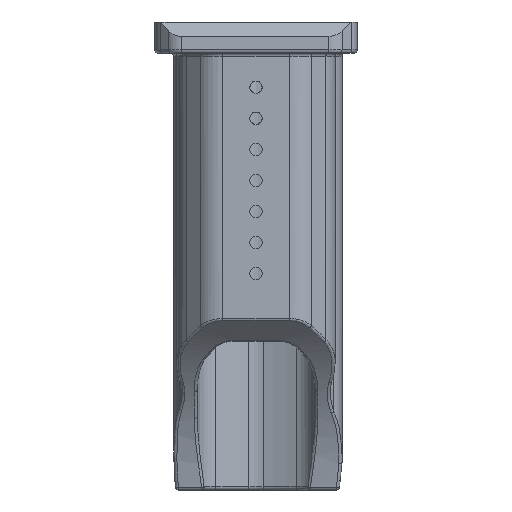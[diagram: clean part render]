
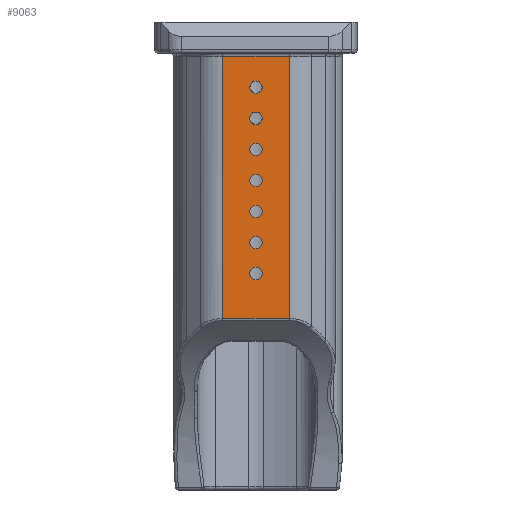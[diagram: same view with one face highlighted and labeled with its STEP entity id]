
A CAD part, front view. The second image highlights one B-rep face of the part: STEP entity #9063.
In plain terms, the highlighted planar face has unit normal (0, -1, 0).
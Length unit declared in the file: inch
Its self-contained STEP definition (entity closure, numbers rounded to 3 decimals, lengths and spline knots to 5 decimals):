
#30=FACE_BOUND('',#1518,.T.);
#31=FACE_BOUND('',#1519,.T.);
#32=FACE_BOUND('',#1520,.T.);
#33=FACE_BOUND('',#1521,.T.);
#34=FACE_BOUND('',#1522,.T.);
#35=FACE_BOUND('',#1523,.T.);
#36=FACE_BOUND('',#1524,.T.);
#308=PLANE('',#9837);
#985=FACE_OUTER_BOUND('',#1517,.T.);
#1517=EDGE_LOOP('',(#7756,#7757,#7758,#7759));
#1518=EDGE_LOOP('',(#7760,#7761));
#1519=EDGE_LOOP('',(#7762,#7763));
#1520=EDGE_LOOP('',(#7764,#7765));
#1521=EDGE_LOOP('',(#7766,#7767));
#1522=EDGE_LOOP('',(#7768,#7769));
#1523=EDGE_LOOP('',(#7770,#7771));
#1524=EDGE_LOOP('',(#7772,#7773));
#2366=LINE('',#16193,#3183);
#2373=LINE('',#16830,#3190);
#2374=LINE('',#16834,#3191);
#2375=LINE('',#16835,#3192);
#3183=VECTOR('',#11880,0.3937);
#3190=VECTOR('',#11945,0.5);
#3191=VECTOR('',#11950,0.3937);
#3192=VECTOR('',#11951,0.3937);
#3409=CIRCLE('',#9371,0.09843);
#3410=CIRCLE('',#9372,0.09843);
#3412=CIRCLE('',#9375,0.09843);
#3413=CIRCLE('',#9376,0.09843);
#3415=CIRCLE('',#9379,0.09843);
#3416=CIRCLE('',#9380,0.09843);
#3418=CIRCLE('',#9383,0.09843);
#3419=CIRCLE('',#9384,0.09843);
#3421=CIRCLE('',#9387,0.09843);
#3422=CIRCLE('',#9388,0.09843);
#3423=CIRCLE('',#9392,0.09843);
#3424=CIRCLE('',#9393,0.09843);
#3427=CIRCLE('',#9398,0.09843);
#3428=CIRCLE('',#9399,0.09843);
#3825=VERTEX_POINT('',#13624);
#3826=VERTEX_POINT('',#13625);
#3828=VERTEX_POINT('',#13632);
#3829=VERTEX_POINT('',#13633);
#3831=VERTEX_POINT('',#13640);
#3832=VERTEX_POINT('',#13641);
#3834=VERTEX_POINT('',#13648);
#3835=VERTEX_POINT('',#13649);
#3837=VERTEX_POINT('',#13656);
#3838=VERTEX_POINT('',#13657);
#3841=VERTEX_POINT('',#13666);
#3842=VERTEX_POINT('',#13667);
#3846=VERTEX_POINT('',#13678);
#3847=VERTEX_POINT('',#13679);
#4361=VERTEX_POINT('',#16170);
#4363=VERTEX_POINT('',#16191);
#4395=VERTEX_POINT('',#16829);
#4396=VERTEX_POINT('',#16833);
#4716=EDGE_CURVE('',#3825,#3826,#3409,.T.);
#4717=EDGE_CURVE('',#3826,#3825,#3410,.T.);
#4720=EDGE_CURVE('',#3828,#3829,#3412,.T.);
#4721=EDGE_CURVE('',#3829,#3828,#3413,.T.);
#4724=EDGE_CURVE('',#3831,#3832,#3415,.T.);
#4725=EDGE_CURVE('',#3832,#3831,#3416,.T.);
#4728=EDGE_CURVE('',#3834,#3835,#3418,.T.);
#4729=EDGE_CURVE('',#3835,#3834,#3419,.T.);
#4732=EDGE_CURVE('',#3837,#3838,#3421,.T.);
#4733=EDGE_CURVE('',#3838,#3837,#3422,.T.);
#4737=EDGE_CURVE('',#3841,#3842,#3423,.T.);
#4738=EDGE_CURVE('',#3842,#3841,#3424,.T.);
#4743=EDGE_CURVE('',#3846,#3847,#3427,.T.);
#4744=EDGE_CURVE('',#3847,#3846,#3428,.T.);
#5540=EDGE_CURVE('',#4363,#4361,#2366,.T.);
#5593=EDGE_CURVE('',#4395,#4361,#2373,.T.);
#5595=EDGE_CURVE('',#4396,#4363,#2374,.T.);
#5596=EDGE_CURVE('',#4395,#4396,#2375,.T.);
#7756=ORIENTED_EDGE('',*,*,#5540,.F.);
#7757=ORIENTED_EDGE('',*,*,#5595,.F.);
#7758=ORIENTED_EDGE('',*,*,#5596,.F.);
#7759=ORIENTED_EDGE('',*,*,#5593,.T.);
#7760=ORIENTED_EDGE('',*,*,#4716,.T.);
#7761=ORIENTED_EDGE('',*,*,#4717,.T.);
#7762=ORIENTED_EDGE('',*,*,#4720,.T.);
#7763=ORIENTED_EDGE('',*,*,#4721,.T.);
#7764=ORIENTED_EDGE('',*,*,#4724,.T.);
#7765=ORIENTED_EDGE('',*,*,#4725,.T.);
#7766=ORIENTED_EDGE('',*,*,#4728,.T.);
#7767=ORIENTED_EDGE('',*,*,#4729,.T.);
#7768=ORIENTED_EDGE('',*,*,#4732,.T.);
#7769=ORIENTED_EDGE('',*,*,#4733,.T.);
#7770=ORIENTED_EDGE('',*,*,#4737,.T.);
#7771=ORIENTED_EDGE('',*,*,#4738,.T.);
#7772=ORIENTED_EDGE('',*,*,#4743,.T.);
#7773=ORIENTED_EDGE('',*,*,#4744,.T.);
#9063=ADVANCED_FACE('',(#985,#30,#31,#32,#33,#34,#35,#36),#308,.T.);
#9371=AXIS2_PLACEMENT_3D('',#13626,#10412,#10413);
#9372=AXIS2_PLACEMENT_3D('',#13627,#10414,#10415);
#9375=AXIS2_PLACEMENT_3D('',#13634,#10421,#10422);
#9376=AXIS2_PLACEMENT_3D('',#13635,#10423,#10424);
#9379=AXIS2_PLACEMENT_3D('',#13642,#10430,#10431);
#9380=AXIS2_PLACEMENT_3D('',#13643,#10432,#10433);
#9383=AXIS2_PLACEMENT_3D('',#13650,#10439,#10440);
#9384=AXIS2_PLACEMENT_3D('',#13651,#10441,#10442);
#9387=AXIS2_PLACEMENT_3D('',#13658,#10448,#10449);
#9388=AXIS2_PLACEMENT_3D('',#13659,#10450,#10451);
#9392=AXIS2_PLACEMENT_3D('',#13668,#10459,#10460);
#9393=AXIS2_PLACEMENT_3D('',#13669,#10461,#10462);
#9398=AXIS2_PLACEMENT_3D('',#13680,#10472,#10473);
#9399=AXIS2_PLACEMENT_3D('',#13681,#10474,#10475);
#9837=AXIS2_PLACEMENT_3D('',#16832,#11948,#11949);
#10412=DIRECTION('center_axis',(0.,1.,0.));
#10413=DIRECTION('ref_axis',(1.,0.,0.));
#10414=DIRECTION('center_axis',(0.,1.,0.));
#10415=DIRECTION('ref_axis',(1.,0.,0.));
#10421=DIRECTION('center_axis',(0.,1.,0.));
#10422=DIRECTION('ref_axis',(1.,0.,0.));
#10423=DIRECTION('center_axis',(0.,1.,0.));
#10424=DIRECTION('ref_axis',(1.,0.,0.));
#10430=DIRECTION('center_axis',(0.,1.,0.));
#10431=DIRECTION('ref_axis',(1.,0.,0.));
#10432=DIRECTION('center_axis',(0.,1.,0.));
#10433=DIRECTION('ref_axis',(1.,0.,0.));
#10439=DIRECTION('center_axis',(0.,1.,0.));
#10440=DIRECTION('ref_axis',(1.,0.,0.));
#10441=DIRECTION('center_axis',(0.,1.,0.));
#10442=DIRECTION('ref_axis',(1.,0.,0.));
#10448=DIRECTION('center_axis',(0.,1.,0.));
#10449=DIRECTION('ref_axis',(1.,0.,0.));
#10450=DIRECTION('center_axis',(0.,1.,0.));
#10451=DIRECTION('ref_axis',(1.,0.,0.));
#10459=DIRECTION('center_axis',(0.,1.,0.));
#10460=DIRECTION('ref_axis',(1.,0.,0.));
#10461=DIRECTION('center_axis',(0.,1.,0.));
#10462=DIRECTION('ref_axis',(1.,0.,0.));
#10472=DIRECTION('center_axis',(0.,1.,0.));
#10473=DIRECTION('ref_axis',(1.,0.,0.));
#10474=DIRECTION('center_axis',(0.,1.,0.));
#10475=DIRECTION('ref_axis',(1.,0.,0.));
#11880=DIRECTION('',(-1.,0.,0.));
#11945=DIRECTION('',(0.,0.,-1.));
#11948=DIRECTION('center_axis',(0.,-1.,0.));
#11949=DIRECTION('ref_axis',(-1.,0.,0.));
#11950=DIRECTION('',(0.,0.,-1.));
#11951=DIRECTION('',(1.,0.,0.));
#13624=CARTESIAN_POINT('',(4.51516,-0.4932,-2.55));
#13625=CARTESIAN_POINT('',(4.31831,-0.4932,-2.55));
#13626=CARTESIAN_POINT('Origin',(4.41673,-0.4932,-2.55));
#13627=CARTESIAN_POINT('Origin',(4.41673,-0.4932,-2.55));
#13632=CARTESIAN_POINT('',(4.51516,-0.4932,-1.55));
#13633=CARTESIAN_POINT('',(4.31831,-0.4932,-1.55));
#13634=CARTESIAN_POINT('Origin',(4.41673,-0.4932,-1.55));
#13635=CARTESIAN_POINT('Origin',(4.41673,-0.4932,-1.55));
#13640=CARTESIAN_POINT('',(4.51516,-0.4932,-2.05));
#13641=CARTESIAN_POINT('',(4.31831,-0.4932,-2.05));
#13642=CARTESIAN_POINT('Origin',(4.41673,-0.4932,-2.05));
#13643=CARTESIAN_POINT('Origin',(4.41673,-0.4932,-2.05));
#13648=CARTESIAN_POINT('',(4.51516,-0.4932,-3.05));
#13649=CARTESIAN_POINT('',(4.31831,-0.4932,-3.05));
#13650=CARTESIAN_POINT('Origin',(4.41673,-0.4932,-3.05));
#13651=CARTESIAN_POINT('Origin',(4.41673,-0.4932,-3.05));
#13656=CARTESIAN_POINT('',(4.51516,-0.4932,-0.55));
#13657=CARTESIAN_POINT('',(4.31831,-0.4932,-0.55));
#13658=CARTESIAN_POINT('Origin',(4.41673,-0.4932,-0.55));
#13659=CARTESIAN_POINT('Origin',(4.41673,-0.4932,-0.55));
#13666=CARTESIAN_POINT('',(4.51516,-0.4932,-1.05));
#13667=CARTESIAN_POINT('',(4.31831,-0.4932,-1.05));
#13668=CARTESIAN_POINT('Origin',(4.41673,-0.4932,-1.05));
#13669=CARTESIAN_POINT('Origin',(4.41673,-0.4932,-1.05));
#13678=CARTESIAN_POINT('',(4.51516,-0.4932,-3.55));
#13679=CARTESIAN_POINT('',(4.31831,-0.4932,-3.55));
#13680=CARTESIAN_POINT('Origin',(4.41673,-0.4932,-3.55));
#13681=CARTESIAN_POINT('Origin',(4.41673,-0.4932,-3.55));
#16170=CARTESIAN_POINT('',(3.87842,-0.4932,-4.27362));
#16191=CARTESIAN_POINT('',(4.95505,-0.4932,-4.27362));
#16193=CARTESIAN_POINT('',(4.95505,-0.4932,-4.27362));
#16829=CARTESIAN_POINT('',(3.87842,-0.4932,-0.05));
#16830=CARTESIAN_POINT('',(3.87842,-0.4932,0.));
#16832=CARTESIAN_POINT('Origin',(5.16216,-0.4932,0.));
#16833=CARTESIAN_POINT('',(4.95505,-0.4932,-0.05));
#16834=CARTESIAN_POINT('',(4.95505,-0.4932,0.));
#16835=CARTESIAN_POINT('',(4.78942,-0.4932,-0.05));
